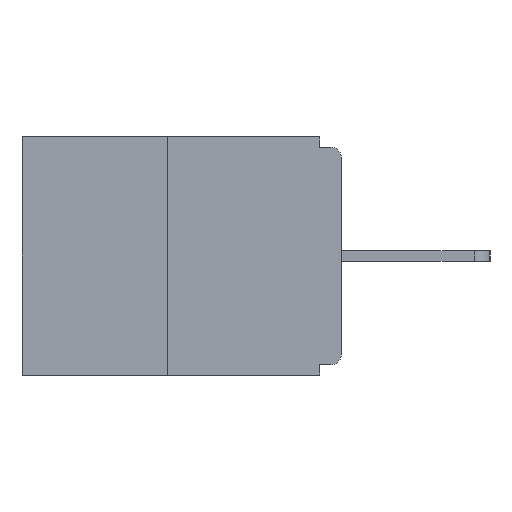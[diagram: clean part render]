
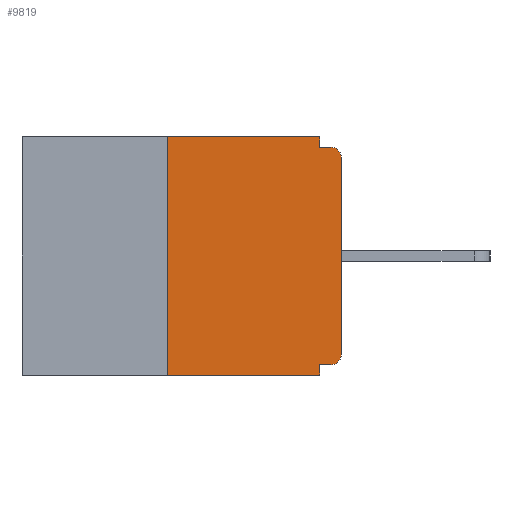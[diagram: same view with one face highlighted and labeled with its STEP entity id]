
A CAD part, left-side view. The second image highlights one B-rep face of the part: STEP entity #9819.
In plain terms, the highlighted planar face has unit normal (-1, 0, 0).
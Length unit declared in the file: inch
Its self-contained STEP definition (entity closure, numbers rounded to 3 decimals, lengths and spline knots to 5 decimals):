
#307 = DIRECTION ( 'NONE',  ( 0., 0., -1. ) ) ;
#336 = DIRECTION ( 'NONE',  ( -1., 0., 0. ) ) ;
#437 = CARTESIAN_POINT ( 'NONE',  ( 0., 0.015, -0.313 ) ) ;
#537 = DIRECTION ( 'NONE',  ( 0., 0., 1. ) ) ;
#708 = VECTOR ( 'NONE', #5626, 39.37008 ) ;
#837 = LINE ( 'NONE', #6504, #13196 ) ;
#888 = PLANE ( 'NONE',  #3992 ) ;
#938 = DIRECTION ( 'NONE',  ( 1., 0., 0. ) ) ;
#1445 = DIRECTION ( 'NONE',  ( 0., -1., 0. ) ) ;
#1505 = ORIENTED_EDGE ( 'NONE', *, *, #2011, .T. ) ;
#1621 = DIRECTION ( 'NONE',  ( 0., 0., -1. ) ) ;
#2011 = EDGE_CURVE ( 'NONE', #10132, #11553, #837, .T. ) ;
#2395 = ORIENTED_EDGE ( 'NONE', *, *, #9622, .T. ) ;
#2493 = EDGE_CURVE ( 'NONE', #10522, #12297, #7002, .T. ) ;
#2559 = LINE ( 'NONE', #11154, #8427 ) ;
#2603 = LINE ( 'NONE', #7233, #14229 ) ;
#2654 = CARTESIAN_POINT ( 'NONE',  ( 0., 0.015, -0.03 ) ) ;
#2785 = EDGE_LOOP ( 'NONE', ( #3727, #11621, #1505, #8067, #13431, #8748, #2395, #4939, #13170, #10364 ) ) ;
#2981 = LINE ( 'NONE', #10732, #14971 ) ;
#3511 = EDGE_CURVE ( 'NONE', #9169, #12297, #11320, .T. ) ;
#3636 = CARTESIAN_POINT ( 'NONE',  ( 0., 0., -0.015 ) ) ;
#3727 = ORIENTED_EDGE ( 'NONE', *, *, #7313, .F. ) ;
#3992 = AXIS2_PLACEMENT_3D ( 'NONE', #9060, #938, #9103 ) ;
#4024 = CIRCLE ( 'NONE', #5293, 0.015 ) ;
#4048 = CARTESIAN_POINT ( 'NONE',  ( 0., 0., 0. ) ) ;
#4662 = EDGE_CURVE ( 'NONE', #7104, #9169, #2559, .T. ) ;
#4939 = ORIENTED_EDGE ( 'NONE', *, *, #2493, .T. ) ;
#5293 = AXIS2_PLACEMENT_3D ( 'NONE', #437, #8603, #1621 ) ;
#5626 = DIRECTION ( 'NONE',  ( 0., 0., -1. ) ) ;
#5716 = CARTESIAN_POINT ( 'NONE',  ( 0., 0.015, -0.328 ) ) ;
#5938 = VECTOR ( 'NONE', #537, 39.37008 ) ;
#6504 = CARTESIAN_POINT ( 'NONE',  ( 0., 0.46, -0.343 ) ) ;
#6898 = CARTESIAN_POINT ( 'NONE',  ( 0., 0.031, -0.328 ) ) ;
#7002 = CIRCLE ( 'NONE', #7537, 0.015 ) ;
#7104 = VERTEX_POINT ( 'NONE', #11445 ) ;
#7233 = CARTESIAN_POINT ( 'NONE',  ( 0., 0.46, 0. ) ) ;
#7248 = CARTESIAN_POINT ( 'NONE',  ( 0., 0.25, -0.343 ) ) ;
#7270 = LINE ( 'NONE', #13704, #708 ) ;
#7313 = EDGE_CURVE ( 'NONE', #10330, #7104, #2603, .T. ) ;
#7537 = AXIS2_PLACEMENT_3D ( 'NONE', #2654, #336, #307 ) ;
#7875 = VECTOR ( 'NONE', #9178, 39.37008 ) ;
#8067 = ORIENTED_EDGE ( 'NONE', *, *, #8955, .F. ) ;
#8317 = CARTESIAN_POINT ( 'NONE',  ( 0., 0.031, -0.015 ) ) ;
#8423 = VERTEX_POINT ( 'NONE', #6898 ) ;
#8427 = VECTOR ( 'NONE', #8711, 39.37008 ) ;
#8603 = DIRECTION ( 'NONE',  ( -1., 0., 0. ) ) ;
#8711 = DIRECTION ( 'NONE',  ( 0., 0., -1. ) ) ;
#8748 = ORIENTED_EDGE ( 'NONE', *, *, #14744, .T. ) ;
#8955 = EDGE_CURVE ( 'NONE', #8423, #11553, #7270, .T. ) ;
#9060 = CARTESIAN_POINT ( 'NONE',  ( 0., 0.46, 0. ) ) ;
#9103 = DIRECTION ( 'NONE',  ( 0., 0., -1. ) ) ;
#9169 = VERTEX_POINT ( 'NONE', #8317 ) ;
#9178 = DIRECTION ( 'NONE',  ( 0., -1., 0. ) ) ;
#9622 = EDGE_CURVE ( 'NONE', #14741, #10522, #13230, .T. ) ;
#9819 = ADVANCED_FACE ( 'NONE', ( #13412 ), #888, .F. ) ;
#9898 = CARTESIAN_POINT ( 'NONE',  ( 0., 0.25, 0. ) ) ;
#10132 = VERTEX_POINT ( 'NONE', #7248 ) ;
#10330 = VERTEX_POINT ( 'NONE', #9898 ) ;
#10364 = ORIENTED_EDGE ( 'NONE', *, *, #4662, .F. ) ;
#10522 = VERTEX_POINT ( 'NONE', #13807 ) ;
#10662 = VERTEX_POINT ( 'NONE', #5716 ) ;
#10732 = CARTESIAN_POINT ( 'NONE',  ( 0., 0., -0.328 ) ) ;
#11154 = CARTESIAN_POINT ( 'NONE',  ( 0., 0.031, 0. ) ) ;
#11320 = LINE ( 'NONE', #3636, #7875 ) ;
#11445 = CARTESIAN_POINT ( 'NONE',  ( 0., 0.031, 0. ) ) ;
#11553 = VERTEX_POINT ( 'NONE', #14565 ) ;
#11621 = ORIENTED_EDGE ( 'NONE', *, *, #14827, .F. ) ;
#11985 = EDGE_CURVE ( 'NONE', #10662, #8423, #2981, .T. ) ;
#12019 = CARTESIAN_POINT ( 'NONE',  ( 0., 0., -0.313 ) ) ;
#12175 = DIRECTION ( 'NONE',  ( 0., 0., 1. ) ) ;
#12297 = VERTEX_POINT ( 'NONE', #13065 ) ;
#12484 = LINE ( 'NONE', #14441, #5938 ) ;
#13055 = DIRECTION ( 'NONE',  ( 0., 1., 0. ) ) ;
#13065 = CARTESIAN_POINT ( 'NONE',  ( 0., 0.015, -0.015 ) ) ;
#13170 = ORIENTED_EDGE ( 'NONE', *, *, #3511, .F. ) ;
#13196 = VECTOR ( 'NONE', #14234, 39.37008 ) ;
#13230 = LINE ( 'NONE', #4048, #13592 ) ;
#13412 = FACE_OUTER_BOUND ( 'NONE', #2785, .T. ) ;
#13431 = ORIENTED_EDGE ( 'NONE', *, *, #11985, .F. ) ;
#13592 = VECTOR ( 'NONE', #12175, 39.37008 ) ;
#13704 = CARTESIAN_POINT ( 'NONE',  ( 0., 0.031, -0.343 ) ) ;
#13807 = CARTESIAN_POINT ( 'NONE',  ( 0., 0., -0.03 ) ) ;
#14229 = VECTOR ( 'NONE', #1445, 39.37008 ) ;
#14234 = DIRECTION ( 'NONE',  ( 0., -1., 0. ) ) ;
#14441 = CARTESIAN_POINT ( 'NONE',  ( 0., 0.25, 0. ) ) ;
#14565 = CARTESIAN_POINT ( 'NONE',  ( 0., 0.031, -0.343 ) ) ;
#14741 = VERTEX_POINT ( 'NONE', #12019 ) ;
#14744 = EDGE_CURVE ( 'NONE', #10662, #14741, #4024, .T. ) ;
#14827 = EDGE_CURVE ( 'NONE', #10132, #10330, #12484, .T. ) ;
#14971 = VECTOR ( 'NONE', #13055, 39.37008 ) ;
